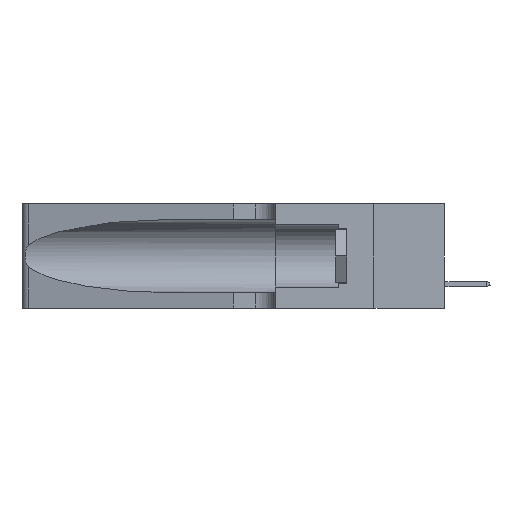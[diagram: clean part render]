
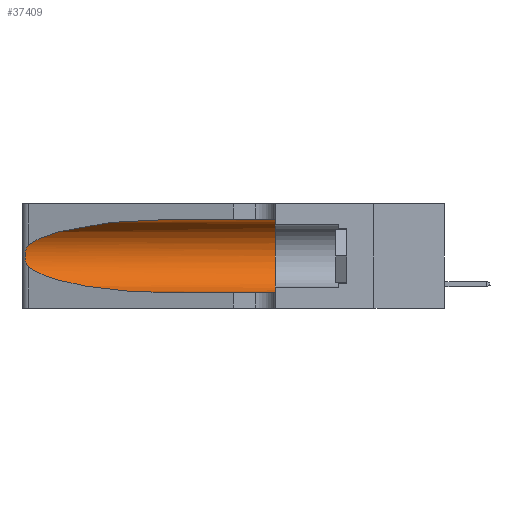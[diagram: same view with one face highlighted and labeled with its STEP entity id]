
A CAD part, left-side view. The second image highlights one B-rep face of the part: STEP entity #37409.
In plain terms, the highlighted cylindrical face has radius 3.308 mm (diameter 6.617 mm), a partial arc.
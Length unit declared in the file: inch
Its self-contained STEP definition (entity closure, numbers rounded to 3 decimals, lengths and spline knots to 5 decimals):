
#598 = CARTESIAN_POINT ( 'NONE',  ( 0.25787, 1.23484, 0.2124 ) ) ;
#667 = CARTESIAN_POINT ( 'NONE',  ( 0.25487, 1.22718, 0.22369 ) ) ;
#779 = EDGE_CURVE ( 'NONE', #33951, #18003, #10117, .T. ) ;
#3407 = CARTESIAN_POINT ( 'NONE',  ( 0.25487, 1.22718, 0.14631 ) ) ;
#3554 = CARTESIAN_POINT ( 'NONE',  ( 0.1305, 1.61858, 0.05475 ) ) ;
#3662 = EDGE_CURVE ( 'NONE', #10681, #41689, #25736, .T. ) ;
#3913 = VECTOR ( 'NONE', #24446, 39.37008 ) ;
#5470 = B_SPLINE_CURVE_WITH_KNOTS ( 'NONE', 3,
 ( #40856, #27487, #44166, #598, #37831, #17925, #24794, #14066, #14654, #20776, #24336, #21165, #21270, #26779 ),
 .UNSPECIFIED., .F., .F.,
 ( 4, 2, 2, 2, 2, 2, 4 ),
 ( 0., 0.00027, 0.00053, 0.00107, 0.0016, 0.00187, 0.00214 ),
 .UNSPECIFIED. ) ;
#7380 = EDGE_CURVE ( 'NONE', #14792, #33951, #5470, .T. ) ;
#8228 = CARTESIAN_POINT ( 'NONE',  ( 0.2373, 1.15595, 0.28018 ) ) ;
#8490 = CARTESIAN_POINT ( 'NONE',  ( 0.1305, 0.72297, 0.31525 ) ) ;
#9082 = CARTESIAN_POINT ( 'NONE',  ( 0.2373, 1.15595, 0.08982 ) ) ;
#9391 = CARTESIAN_POINT ( 'NONE',  ( 0.1305, 0.35, 0.05475 ) ) ;
#9717 = DIRECTION ( 'NONE',  ( 0., -1., 0. ) ) ;
#10117 =( BOUNDED_CURVE ( )  B_SPLINE_CURVE ( 3, ( #28912, #9082, #25957, #39852 ),
 .UNSPECIFIED., .F., .F. ) 
 B_SPLINE_CURVE_WITH_KNOTS ( ( 4, 4 ),
 ( 3.44316, 4.71239 ),
 .UNSPECIFIED. ) 
 CURVE ( )  GEOMETRIC_REPRESENTATION_ITEM ( )  RATIONAL_B_SPLINE_CURVE ( ( 1., 0.87, 0.87, 1. ) ) 
 REPRESENTATION_ITEM ( '' )  );
#10681 = VERTEX_POINT ( 'NONE', #42073 ) ;
#10933 = EDGE_CURVE ( 'NONE', #18003, #41689, #40326, .T. ) ;
#11314 = EDGE_LOOP ( 'NONE', ( #30966, #42429, #38500, #15487, #29795, #32389 ) ) ;
#11688 = CARTESIAN_POINT ( 'NONE',  ( 0.25487, 1.22718, 0.22369 ) ) ;
#12284 = CARTESIAN_POINT ( 'NONE',  ( 0.1305, 1.61858, 0.31525 ) ) ;
#12603 = DIRECTION ( 'NONE',  ( 0., 1., 0. ) ) ;
#14066 = CARTESIAN_POINT ( 'NONE',  ( 0.26075, 1.23896, 0.178 ) ) ;
#14654 = CARTESIAN_POINT ( 'NONE',  ( 0.26017, 1.23833, 0.17102 ) ) ;
#14792 = VERTEX_POINT ( 'NONE', #667 ) ;
#15251 = DIRECTION ( 'NONE',  ( 0., -1., 0. ) ) ;
#15487 = ORIENTED_EDGE ( 'NONE', *, *, #10933, .T. ) ;
#17490 =( BOUNDED_CURVE ( )  B_SPLINE_CURVE ( 3, ( #38867, #31800, #8228, #11688 ),
 .UNSPECIFIED., .F., .F. ) 
 B_SPLINE_CURVE_WITH_KNOTS ( ( 4, 4 ),
 ( 1.5708, 2.84003 ),
 .UNSPECIFIED. ) 
 CURVE ( )  GEOMETRIC_REPRESENTATION_ITEM ( )  RATIONAL_B_SPLINE_CURVE ( ( 1., 0.87, 0.87, 1. ) ) 
 REPRESENTATION_ITEM ( '' )  );
#17768 = DIRECTION ( 'NONE',  ( 0., 0., 1. ) ) ;
#17925 = CARTESIAN_POINT ( 'NONE',  ( 0.26018, 1.23835, 0.19895 ) ) ;
#18003 = VERTEX_POINT ( 'NONE', #18053 ) ;
#18053 = CARTESIAN_POINT ( 'NONE',  ( 0.1305, 0.72297, 0.05475 ) ) ;
#20776 = CARTESIAN_POINT ( 'NONE',  ( 0.25856, 1.23593, 0.16098 ) ) ;
#21165 = CARTESIAN_POINT ( 'NONE',  ( 0.25639, 1.23186, 0.15144 ) ) ;
#21270 = CARTESIAN_POINT ( 'NONE',  ( 0.25555, 1.22993, 0.14849 ) ) ;
#23015 = AXIS2_PLACEMENT_3D ( 'NONE', #43384, #9717, #30008 ) ;
#24336 = CARTESIAN_POINT ( 'NONE',  ( 0.25789, 1.23486, 0.15765 ) ) ;
#24446 = DIRECTION ( 'NONE',  ( 0., -1., 0. ) ) ;
#24794 = CARTESIAN_POINT ( 'NONE',  ( 0.26075, 1.23896, 0.19203 ) ) ;
#25736 = CIRCLE ( 'NONE', #42231, 0.13025 ) ;
#25957 = CARTESIAN_POINT ( 'NONE',  ( 0.18966, 0.96281, 0.05475 ) ) ;
#26779 = CARTESIAN_POINT ( 'NONE',  ( 0.25487, 1.22718, 0.14631 ) ) ;
#27487 = CARTESIAN_POINT ( 'NONE',  ( 0.25555, 1.22994, 0.2215 ) ) ;
#27936 = VERTEX_POINT ( 'NONE', #8490 ) ;
#28062 = LINE ( 'NONE', #12284, #30674 ) ;
#28912 = CARTESIAN_POINT ( 'NONE',  ( 0.25487, 1.22718, 0.14631 ) ) ;
#29795 = ORIENTED_EDGE ( 'NONE', *, *, #3662, .F. ) ;
#30008 = DIRECTION ( 'NONE',  ( 0., 0., -1. ) ) ;
#30674 = VECTOR ( 'NONE', #15251, 39.37008 ) ;
#30966 = ORIENTED_EDGE ( 'NONE', *, *, #33204, .T. ) ;
#31800 = CARTESIAN_POINT ( 'NONE',  ( 0.18966, 0.96281, 0.31525 ) ) ;
#32389 = ORIENTED_EDGE ( 'NONE', *, *, #33844, .F. ) ;
#32755 = CYLINDRICAL_SURFACE ( 'NONE', #23015, 0.13025 ) ;
#33204 = EDGE_CURVE ( 'NONE', #27936, #14792, #17490, .T. ) ;
#33844 = EDGE_CURVE ( 'NONE', #27936, #10681, #28062, .T. ) ;
#33951 = VERTEX_POINT ( 'NONE', #3407 ) ;
#34896 = FACE_OUTER_BOUND ( 'NONE', #11314, .T. ) ;
#37409 = ADVANCED_FACE ( 'NONE', ( #34896 ), #32755, .F. ) ;
#37831 = CARTESIAN_POINT ( 'NONE',  ( 0.25854, 1.2359, 0.20912 ) ) ;
#38500 = ORIENTED_EDGE ( 'NONE', *, *, #779, .T. ) ;
#38867 = CARTESIAN_POINT ( 'NONE',  ( 0.1305, 0.72297, 0.31525 ) ) ;
#39852 = CARTESIAN_POINT ( 'NONE',  ( 0.1305, 0.72297, 0.05475 ) ) ;
#40326 = LINE ( 'NONE', #3554, #3913 ) ;
#40839 = CARTESIAN_POINT ( 'NONE',  ( 0.1305, 0.35, 0.185 ) ) ;
#40856 = CARTESIAN_POINT ( 'NONE',  ( 0.25487, 1.22718, 0.22369 ) ) ;
#41689 = VERTEX_POINT ( 'NONE', #9391 ) ;
#42073 = CARTESIAN_POINT ( 'NONE',  ( 0.1305, 0.35, 0.31525 ) ) ;
#42231 = AXIS2_PLACEMENT_3D ( 'NONE', #40839, #12603, #17768 ) ;
#42429 = ORIENTED_EDGE ( 'NONE', *, *, #7380, .T. ) ;
#43384 = CARTESIAN_POINT ( 'NONE',  ( 0.1305, 1.61858, 0.185 ) ) ;
#44166 = CARTESIAN_POINT ( 'NONE',  ( 0.25639, 1.23184, 0.21858 ) ) ;
